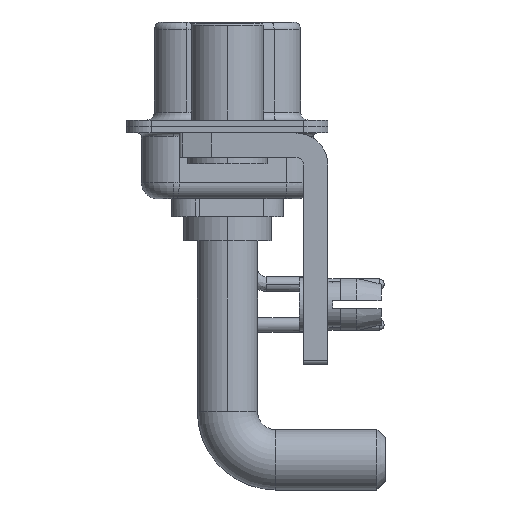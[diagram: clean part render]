
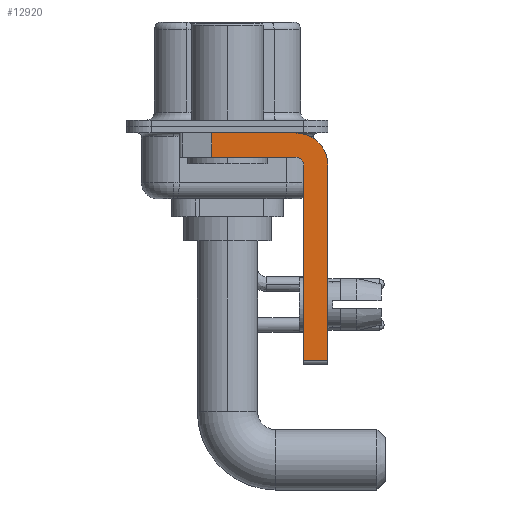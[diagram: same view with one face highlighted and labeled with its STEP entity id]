
A CAD part, left-side view. The second image highlights one B-rep face of the part: STEP entity #12920.
In plain terms, the highlighted planar face has unit normal (-1, 0, 0).
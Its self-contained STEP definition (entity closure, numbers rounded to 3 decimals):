
#328 = VECTOR ( 'NONE', #29142, 1000. ) ;
#351 = AXIS2_PLACEMENT_3D ( 'NONE', #28020, #18112, #25103 ) ;
#597 = CARTESIAN_POINT ( 'NONE',  ( -2.9, 3., -0.4 ) ) ;
#619 = CARTESIAN_POINT ( 'NONE',  ( -2.9, -4.25, -14.55 ) ) ;
#1212 = DIRECTION ( 'NONE',  ( 0., 0., 1. ) ) ;
#1373 = DIRECTION ( 'NONE',  ( -1., 0., 0. ) ) ;
#1504 = EDGE_LOOP ( 'NONE', ( #2546, #15170, #27822, #1537, #15326, #26363, #20974, #2469 ) ) ;
#1537 = ORIENTED_EDGE ( 'NONE', *, *, #15227, .F. ) ;
#2070 = DIRECTION ( 'NONE',  ( 0., 0., -1. ) ) ;
#2469 = ORIENTED_EDGE ( 'NONE', *, *, #21230, .F. ) ;
#2546 = ORIENTED_EDGE ( 'NONE', *, *, #21986, .F. ) ;
#4315 = DIRECTION ( 'NONE',  ( 0., 1., 0. ) ) ;
#5087 = AXIS2_PLACEMENT_3D ( 'NONE', #21144, #1373, #1212 ) ;
#5987 = LINE ( 'NONE', #15840, #328 ) ;
#9276 = VECTOR ( 'NONE', #27676, 1000. ) ;
#9521 = CIRCLE ( 'NONE', #29123, 2. ) ;
#10517 = DIRECTION ( 'NONE',  ( 0., -1., 0. ) ) ;
#10763 = CIRCLE ( 'NONE', #5087, 0.5 ) ;
#11824 = VECTOR ( 'NONE', #4315, 1000. ) ;
#12060 = CARTESIAN_POINT ( 'NONE',  ( -2.9, -4.25, -1.9 ) ) ;
#12347 = VERTEX_POINT ( 'NONE', #17925 ) ;
#12791 = CARTESIAN_POINT ( 'NONE',  ( -2.9, 0.978, -0.4 ) ) ;
#12920 = ADVANCED_FACE ( 'NONE', ( #17635 ), #27540, .F. ) ;
#12986 = CARTESIAN_POINT ( 'NONE',  ( -2.9, -6.25, -2.4 ) ) ;
#13027 = VERTEX_POINT ( 'NONE', #24779 ) ;
#13041 = EDGE_CURVE ( 'NONE', #26995, #27543, #27373, .T. ) ;
#13484 = EDGE_CURVE ( 'NONE', #26995, #13540, #5987, .T. ) ;
#13512 = VECTOR ( 'NONE', #2070, 1000. ) ;
#13540 = VERTEX_POINT ( 'NONE', #14677 ) ;
#14475 = CARTESIAN_POINT ( 'NONE',  ( -2.9, 0.978, -1.9 ) ) ;
#14541 = CARTESIAN_POINT ( 'NONE',  ( -2.9, -4.75, -14.55 ) ) ;
#14677 = CARTESIAN_POINT ( 'NONE',  ( -2.9, -4.75, -2.4 ) ) ;
#15017 = CARTESIAN_POINT ( 'NONE',  ( -2.9, -6.25, -2.4 ) ) ;
#15123 = CARTESIAN_POINT ( 'NONE',  ( -2.9, -6.25, -14.55 ) ) ;
#15170 = ORIENTED_EDGE ( 'NONE', *, *, #18838, .T. ) ;
#15227 = EDGE_CURVE ( 'NONE', #13540, #13027, #10763, .T. ) ;
#15326 = ORIENTED_EDGE ( 'NONE', *, *, #13484, .F. ) ;
#15840 = CARTESIAN_POINT ( 'NONE',  ( -2.9, -4.75, -14.8 ) ) ;
#16908 = LINE ( 'NONE', #14475, #18695 ) ;
#16996 = DIRECTION ( 'NONE',  ( 0., 0., -1. ) ) ;
#17635 = FACE_OUTER_BOUND ( 'NONE', #1504, .T. ) ;
#17925 = CARTESIAN_POINT ( 'NONE',  ( -2.9, 0.978, -1.9 ) ) ;
#17927 = CARTESIAN_POINT ( 'NONE',  ( -2.9, -4.25, -2.4 ) ) ;
#18112 = DIRECTION ( 'NONE',  ( 1., 0., 0. ) ) ;
#18416 = LINE ( 'NONE', #597, #9276 ) ;
#18695 = VECTOR ( 'NONE', #28932, 1000. ) ;
#18838 = EDGE_CURVE ( 'NONE', #28350, #12347, #16908, .T. ) ;
#20919 = VERTEX_POINT ( 'NONE', #12986 ) ;
#20974 = ORIENTED_EDGE ( 'NONE', *, *, #25560, .F. ) ;
#21144 = CARTESIAN_POINT ( 'NONE',  ( -2.9, -4.25, -2.4 ) ) ;
#21230 = EDGE_CURVE ( 'NONE', #23871, #20919, #9521, .T. ) ;
#21456 = EDGE_CURVE ( 'NONE', #13027, #12347, #32013, .T. ) ;
#21986 = EDGE_CURVE ( 'NONE', #28350, #23871, #18416, .T. ) ;
#23871 = VERTEX_POINT ( 'NONE', #26386 ) ;
#24779 = CARTESIAN_POINT ( 'NONE',  ( -2.9, -4.25, -1.9 ) ) ;
#24791 = DIRECTION ( 'NONE',  ( 1., 0., 0. ) ) ;
#25103 = DIRECTION ( 'NONE',  ( 0., 0., -1. ) ) ;
#25560 = EDGE_CURVE ( 'NONE', #20919, #27543, #26716, .T. ) ;
#26363 = ORIENTED_EDGE ( 'NONE', *, *, #13041, .T. ) ;
#26386 = CARTESIAN_POINT ( 'NONE',  ( -2.9, -4.25, -0.4 ) ) ;
#26716 = LINE ( 'NONE', #15017, #13512 ) ;
#26995 = VERTEX_POINT ( 'NONE', #14541 ) ;
#27373 = LINE ( 'NONE', #619, #28338 ) ;
#27540 = PLANE ( 'NONE',  #351 ) ;
#27543 = VERTEX_POINT ( 'NONE', #15123 ) ;
#27676 = DIRECTION ( 'NONE',  ( 0., -1., 0. ) ) ;
#27822 = ORIENTED_EDGE ( 'NONE', *, *, #21456, .F. ) ;
#28020 = CARTESIAN_POINT ( 'NONE',  ( -2.9, -4.25, -2.4 ) ) ;
#28338 = VECTOR ( 'NONE', #10517, 1000. ) ;
#28350 = VERTEX_POINT ( 'NONE', #12791 ) ;
#28932 = DIRECTION ( 'NONE',  ( 0., 0., -1. ) ) ;
#29123 = AXIS2_PLACEMENT_3D ( 'NONE', #17927, #24791, #16996 ) ;
#29142 = DIRECTION ( 'NONE',  ( 0., 0., 1. ) ) ;
#32013 = LINE ( 'NONE', #12060, #11824 ) ;
